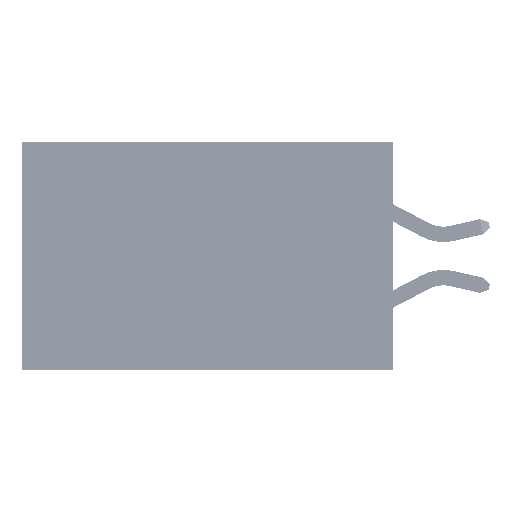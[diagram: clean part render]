
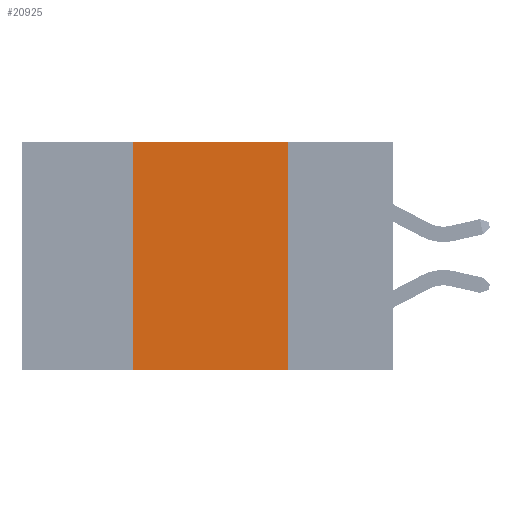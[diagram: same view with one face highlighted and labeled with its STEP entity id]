
A CAD part, left-side view. The second image highlights one B-rep face of the part: STEP entity #20925.
In plain terms, the highlighted planar face has unit normal (-1, 0, 0).
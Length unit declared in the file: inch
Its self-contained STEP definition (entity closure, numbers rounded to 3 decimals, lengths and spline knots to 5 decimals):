
#2985 = LINE ( 'NONE', #22182, #45440 ) ;
#3435 = DIRECTION ( 'NONE',  ( 0., 0., 1. ) ) ;
#3622 = VECTOR ( 'NONE', #40291, 39.37008 ) ;
#4378 = PLANE ( 'NONE',  #4605 ) ;
#4598 = CARTESIAN_POINT ( 'NONE',  ( 0., 0.6, 0. ) ) ;
#4605 = AXIS2_PLACEMENT_3D ( 'NONE', #30222, #26581, #7655 ) ;
#5072 = VERTEX_POINT ( 'NONE', #12711 ) ;
#6169 = CARTESIAN_POINT ( 'NONE',  ( 0., 0.42, -0.37 ) ) ;
#6182 = CARTESIAN_POINT ( 'NONE',  ( 0., 0.17, 0. ) ) ;
#7655 = DIRECTION ( 'NONE',  ( 0., 0., -1. ) ) ;
#9047 = LINE ( 'NONE', #30978, #19090 ) ;
#10960 = FACE_OUTER_BOUND ( 'NONE', #44269, .T. ) ;
#11639 = DIRECTION ( 'NONE',  ( 0., -1., 0. ) ) ;
#12180 = VECTOR ( 'NONE', #11639, 39.37008 ) ;
#12711 = CARTESIAN_POINT ( 'NONE',  ( 0., 0.42, 0. ) ) ;
#12998 = LINE ( 'NONE', #6182, #3622 ) ;
#13463 = EDGE_CURVE ( 'NONE', #5072, #15371, #41700, .T. ) ;
#13878 = CARTESIAN_POINT ( 'NONE',  ( 0., 0.17, 0. ) ) ;
#15371 = VERTEX_POINT ( 'NONE', #13878 ) ;
#18122 = VERTEX_POINT ( 'NONE', #38320 ) ;
#19090 = VECTOR ( 'NONE', #37940, 39.37008 ) ;
#20925 = ADVANCED_FACE ( 'NONE', ( #10960 ), #4378, .F. ) ;
#22182 = CARTESIAN_POINT ( 'NONE',  ( 0., 0.42, 0. ) ) ;
#26581 = DIRECTION ( 'NONE',  ( 1., 0., 0. ) ) ;
#27033 = EDGE_CURVE ( 'NONE', #15371, #18122, #12998, .T. ) ;
#27761 = ORIENTED_EDGE ( 'NONE', *, *, #27033, .F. ) ;
#30222 = CARTESIAN_POINT ( 'NONE',  ( 0., 0.6, 0. ) ) ;
#30978 = CARTESIAN_POINT ( 'NONE',  ( 0., 0.6, -0.37 ) ) ;
#36363 = EDGE_CURVE ( 'NONE', #40951, #18122, #9047, .T. ) ;
#37707 = ORIENTED_EDGE ( 'NONE', *, *, #38049, .F. ) ;
#37940 = DIRECTION ( 'NONE',  ( 0., -1., 0. ) ) ;
#38049 = EDGE_CURVE ( 'NONE', #40951, #5072, #2985, .T. ) ;
#38320 = CARTESIAN_POINT ( 'NONE',  ( 0., 0.17, -0.37 ) ) ;
#40291 = DIRECTION ( 'NONE',  ( 0., 0., -1. ) ) ;
#40951 = VERTEX_POINT ( 'NONE', #6169 ) ;
#41700 = LINE ( 'NONE', #4598, #12180 ) ;
#44269 = EDGE_LOOP ( 'NONE', ( #27761, #47475, #37707, #48758 ) ) ;
#45440 = VECTOR ( 'NONE', #3435, 39.37008 ) ;
#47475 = ORIENTED_EDGE ( 'NONE', *, *, #13463, .F. ) ;
#48758 = ORIENTED_EDGE ( 'NONE', *, *, #36363, .T. ) ;
